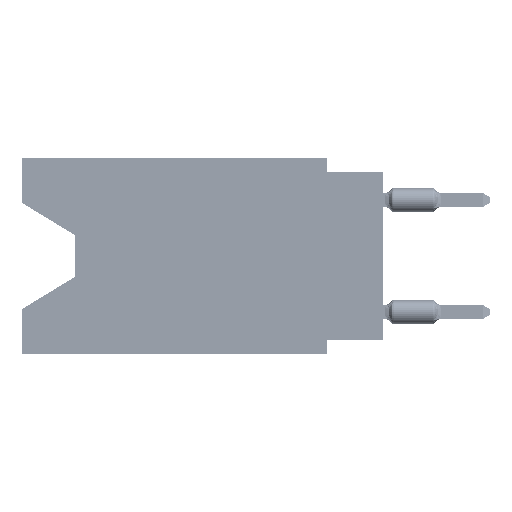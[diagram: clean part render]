
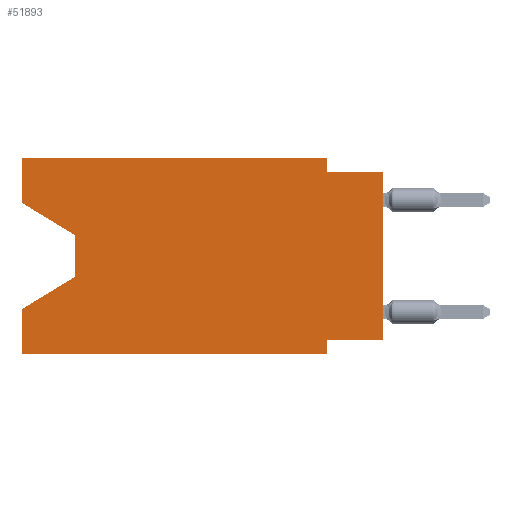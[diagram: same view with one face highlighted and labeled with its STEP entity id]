
A CAD part, left-side view. The second image highlights one B-rep face of the part: STEP entity #51893.
In plain terms, the highlighted planar face has unit normal (-1, 0, 0).
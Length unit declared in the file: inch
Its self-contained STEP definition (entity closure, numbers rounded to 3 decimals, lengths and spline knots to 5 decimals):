
#1635 = CARTESIAN_POINT ( 'NONE',  ( 0., 0.1, -0.025 ) ) ;
#1686 = DIRECTION ( 'NONE',  ( 0., -1., 0. ) ) ;
#3207 = CARTESIAN_POINT ( 'NONE',  ( 0., 0.645, 0. ) ) ;
#3651 = DIRECTION ( 'NONE',  ( 0., -1., 0. ) ) ;
#3698 = DIRECTION ( 'NONE',  ( 0., 0., 1. ) ) ;
#4155 = ORIENTED_EDGE ( 'NONE', *, *, #21464, .T. ) ;
#4907 = CARTESIAN_POINT ( 'NONE',  ( 0., 0.645, -0.35 ) ) ;
#8913 = EDGE_CURVE ( 'NONE', #10704, #68891, #60359, .T. ) ;
#10704 = VERTEX_POINT ( 'NONE', #55377 ) ;
#12636 = LINE ( 'NONE', #64774, #20599 ) ;
#14137 = ORIENTED_EDGE ( 'NONE', *, *, #77022, .T. ) ;
#14566 = CARTESIAN_POINT ( 'NONE',  ( 0., 0., -0.025 ) ) ;
#14822 = CARTESIAN_POINT ( 'NONE',  ( 0., 0.645, -0.35 ) ) ;
#17398 = ORIENTED_EDGE ( 'NONE', *, *, #36460, .T. ) ;
#18442 = LINE ( 'NONE', #4907, #19075 ) ;
#19075 = VECTOR ( 'NONE', #34361, 39.37008 ) ;
#19871 = EDGE_CURVE ( 'NONE', #35043, #29684, #75202, .T. ) ;
#20399 = ORIENTED_EDGE ( 'NONE', *, *, #65018, .F. ) ;
#20599 = VECTOR ( 'NONE', #72027, 39.37008 ) ;
#21464 = EDGE_CURVE ( 'NONE', #10704, #46620, #90285, .T. ) ;
#21536 = LINE ( 'NONE', #80951, #57271 ) ;
#22958 = VECTOR ( 'NONE', #49518, 39.37008 ) ;
#23179 = CARTESIAN_POINT ( 'NONE',  ( 0., 0., -0.325 ) ) ;
#23401 = EDGE_CURVE ( 'NONE', #29168, #71142, #58660, .T. ) ;
#24055 = CARTESIAN_POINT ( 'NONE',  ( 0., 0.55, -0.138 ) ) ;
#25741 = DIRECTION ( 'NONE',  ( 0., -0.855, -0.519 ) ) ;
#26963 = VECTOR ( 'NONE', #3698, 39.37008 ) ;
#27783 = VERTEX_POINT ( 'NONE', #50433 ) ;
#29168 = VERTEX_POINT ( 'NONE', #57694 ) ;
#29684 = VERTEX_POINT ( 'NONE', #80781 ) ;
#30749 = DIRECTION ( 'NONE',  ( 1., 0., 0. ) ) ;
#30981 = VECTOR ( 'NONE', #52283, 39.37008 ) ;
#34225 = CARTESIAN_POINT ( 'NONE',  ( 0., 0.645, 0. ) ) ;
#34361 = DIRECTION ( 'NONE',  ( 0., -1., 0. ) ) ;
#35040 = CARTESIAN_POINT ( 'NONE',  ( 0., 0.1, 0. ) ) ;
#35043 = VERTEX_POINT ( 'NONE', #14822 ) ;
#36460 = EDGE_CURVE ( 'NONE', #71968, #52371, #76448, .T. ) ;
#39533 = DIRECTION ( 'NONE',  ( 0., 0., 1. ) ) ;
#40334 = LINE ( 'NONE', #69822, #49756 ) ;
#46620 = VERTEX_POINT ( 'NONE', #14566 ) ;
#46929 = CARTESIAN_POINT ( 'NONE',  ( 0., 0.55, -0.138 ) ) ;
#47349 = ORIENTED_EDGE ( 'NONE', *, *, #19871, .F. ) ;
#47616 = ORIENTED_EDGE ( 'NONE', *, *, #8913, .F. ) ;
#47967 = AXIS2_PLACEMENT_3D ( 'NONE', #67442, #30749, #60193 ) ;
#48458 = VECTOR ( 'NONE', #25741, 39.37008 ) ;
#49043 = VECTOR ( 'NONE', #63702, 39.37008 ) ;
#49050 = EDGE_LOOP ( 'NONE', ( #17398, #14137, #93150, #47349, #75915, #20399, #47616, #4155, #71042, #93965, #62607, #81876 ) ) ;
#49518 = DIRECTION ( 'NONE',  ( 0., 0., -1. ) ) ;
#49655 = LINE ( 'NONE', #34225, #49043 ) ;
#49756 = VECTOR ( 'NONE', #3651, 39.37008 ) ;
#50433 = CARTESIAN_POINT ( 'NONE',  ( 0., 0.645, 0. ) ) ;
#51893 = ADVANCED_FACE ( 'NONE', ( #62125 ), #54851, .F. ) ;
#52121 = CARTESIAN_POINT ( 'NONE',  ( 0., 0., 0. ) ) ;
#52283 = DIRECTION ( 'NONE',  ( 0., 0., -1. ) ) ;
#52371 = VERTEX_POINT ( 'NONE', #24055 ) ;
#54851 = PLANE ( 'NONE',  #47967 ) ;
#55377 = CARTESIAN_POINT ( 'NONE',  ( 0., 0., -0.325 ) ) ;
#57271 = VECTOR ( 'NONE', #59667, 39.37008 ) ;
#57293 = EDGE_CURVE ( 'NONE', #71142, #46620, #68339, .T. ) ;
#57694 = CARTESIAN_POINT ( 'NONE',  ( 0., 0.1, 0. ) ) ;
#58660 = LINE ( 'NONE', #35040, #22958 ) ;
#59667 = DIRECTION ( 'NONE',  ( 0., 0.855, -0.519 ) ) ;
#60031 = VERTEX_POINT ( 'NONE', #63646 ) ;
#60193 = DIRECTION ( 'NONE',  ( 0., 0., -1. ) ) ;
#60359 = LINE ( 'NONE', #23179, #69558 ) ;
#62125 = FACE_OUTER_BOUND ( 'NONE', #49050, .T. ) ;
#62607 = ORIENTED_EDGE ( 'NONE', *, *, #63861, .F. ) ;
#63646 = CARTESIAN_POINT ( 'NONE',  ( 0., 0.55, -0.212 ) ) ;
#63702 = DIRECTION ( 'NONE',  ( 0., 0., 1. ) ) ;
#63861 = EDGE_CURVE ( 'NONE', #27783, #29168, #40334, .T. ) ;
#64107 = VECTOR ( 'NONE', #1686, 39.37008 ) ;
#64774 = CARTESIAN_POINT ( 'NONE',  ( 0., 0.1, -0.35 ) ) ;
#65018 = EDGE_CURVE ( 'NONE', #68891, #66506, #12636, .T. ) ;
#66506 = VERTEX_POINT ( 'NONE', #80843 ) ;
#67442 = CARTESIAN_POINT ( 'NONE',  ( 0., 0.645, 0. ) ) ;
#68339 = LINE ( 'NONE', #89613, #64107 ) ;
#68558 = CARTESIAN_POINT ( 'NONE',  ( 0., 0.645, -0.08025 ) ) ;
#68891 = VERTEX_POINT ( 'NONE', #82063 ) ;
#69558 = VECTOR ( 'NONE', #74367, 39.37008 ) ;
#69822 = CARTESIAN_POINT ( 'NONE',  ( 0., 0.645, 0. ) ) ;
#71042 = ORIENTED_EDGE ( 'NONE', *, *, #57293, .F. ) ;
#71142 = VERTEX_POINT ( 'NONE', #1635 ) ;
#71968 = VERTEX_POINT ( 'NONE', #68558 ) ;
#72027 = DIRECTION ( 'NONE',  ( 0., 0., -1. ) ) ;
#74367 = DIRECTION ( 'NONE',  ( 0., 1., 0. ) ) ;
#75202 = LINE ( 'NONE', #3207, #26963 ) ;
#75466 = LINE ( 'NONE', #46929, #30981 ) ;
#75915 = ORIENTED_EDGE ( 'NONE', *, *, #81827, .T. ) ;
#76448 = LINE ( 'NONE', #84189, #48458 ) ;
#77022 = EDGE_CURVE ( 'NONE', #52371, #60031, #75466, .T. ) ;
#80781 = CARTESIAN_POINT ( 'NONE',  ( 0., 0.645, -0.26975 ) ) ;
#80843 = CARTESIAN_POINT ( 'NONE',  ( 0., 0.1, -0.35 ) ) ;
#80951 = CARTESIAN_POINT ( 'NONE',  ( 0., 0.55, -0.212 ) ) ;
#81827 = EDGE_CURVE ( 'NONE', #35043, #66506, #18442, .T. ) ;
#81876 = ORIENTED_EDGE ( 'NONE', *, *, #88450, .F. ) ;
#82063 = CARTESIAN_POINT ( 'NONE',  ( 0., 0.1, -0.325 ) ) ;
#84189 = CARTESIAN_POINT ( 'NONE',  ( 0., 0.645, -0.08025 ) ) ;
#88450 = EDGE_CURVE ( 'NONE', #71968, #27783, #49655, .T. ) ;
#89613 = CARTESIAN_POINT ( 'NONE',  ( 0., 0., -0.025 ) ) ;
#90285 = LINE ( 'NONE', #52121, #95093 ) ;
#91579 = EDGE_CURVE ( 'NONE', #60031, #29684, #21536, .T. ) ;
#93150 = ORIENTED_EDGE ( 'NONE', *, *, #91579, .T. ) ;
#93965 = ORIENTED_EDGE ( 'NONE', *, *, #23401, .F. ) ;
#95093 = VECTOR ( 'NONE', #39533, 39.37008 ) ;
